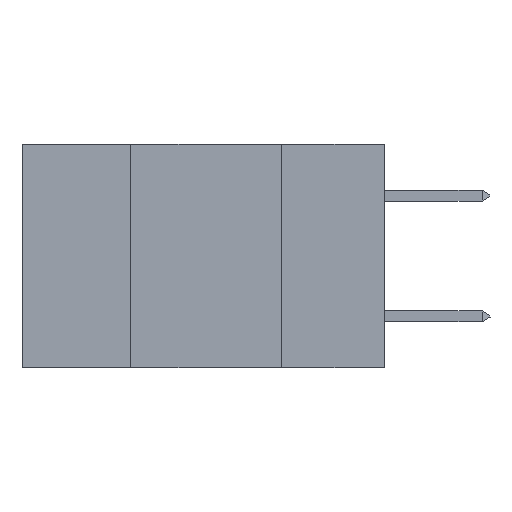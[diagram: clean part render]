
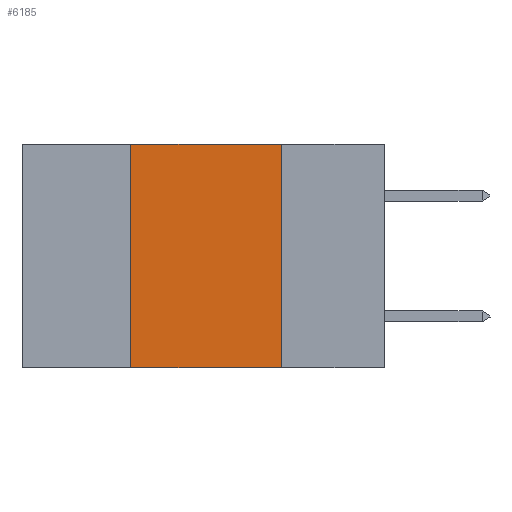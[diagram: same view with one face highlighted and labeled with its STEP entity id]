
A CAD part, left-side view. The second image highlights one B-rep face of the part: STEP entity #6185.
In plain terms, the highlighted planar face has unit normal (-1, 0, 0).
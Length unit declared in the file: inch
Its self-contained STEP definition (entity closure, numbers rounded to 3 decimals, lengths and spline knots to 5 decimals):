
#1363 = EDGE_CURVE ( 'NONE', #12753, #10109, #22118, .T. ) ;
#2100 = CARTESIAN_POINT ( 'NONE',  ( 0., 0.17, 0. ) ) ;
#2631 = DIRECTION ( 'NONE',  ( 1., 0., 0. ) ) ;
#4251 = VECTOR ( 'NONE', #13621, 39.37008 ) ;
#4387 = ORIENTED_EDGE ( 'NONE', *, *, #22126, .F. ) ;
#5815 = ORIENTED_EDGE ( 'NONE', *, *, #17179, .F. ) ;
#6185 = ADVANCED_FACE ( 'NONE', ( #22213 ), #7156, .F. ) ;
#7050 = DIRECTION ( 'NONE',  ( 0., -1., 0. ) ) ;
#7156 = PLANE ( 'NONE',  #24758 ) ;
#8880 = VERTEX_POINT ( 'NONE', #9145 ) ;
#9145 = CARTESIAN_POINT ( 'NONE',  ( 0., 0.42, 0. ) ) ;
#9714 = CARTESIAN_POINT ( 'NONE',  ( 0., 0.17, 0. ) ) ;
#10109 = VERTEX_POINT ( 'NONE', #13643 ) ;
#10728 = LINE ( 'NONE', #18353, #13745 ) ;
#11104 = CARTESIAN_POINT ( 'NONE',  ( 0., 0.6, -0.37 ) ) ;
#11514 = ORIENTED_EDGE ( 'NONE', *, *, #1363, .F. ) ;
#12753 = VERTEX_POINT ( 'NONE', #9714 ) ;
#13314 = VECTOR ( 'NONE', #19285, 39.37008 ) ;
#13621 = DIRECTION ( 'NONE',  ( 0., -1., 0. ) ) ;
#13643 = CARTESIAN_POINT ( 'NONE',  ( 0., 0.17, -0.37 ) ) ;
#13745 = VECTOR ( 'NONE', #27083, 39.37008 ) ;
#15365 = ORIENTED_EDGE ( 'NONE', *, *, #23207, .T. ) ;
#15604 = VECTOR ( 'NONE', #7050, 39.37008 ) ;
#17179 = EDGE_CURVE ( 'NONE', #8880, #12753, #18447, .T. ) ;
#18353 = CARTESIAN_POINT ( 'NONE',  ( 0., 0.42, 0. ) ) ;
#18447 = LINE ( 'NONE', #19902, #4251 ) ;
#19285 = DIRECTION ( 'NONE',  ( 0., 0., -1. ) ) ;
#19902 = CARTESIAN_POINT ( 'NONE',  ( 0., 0.6, 0. ) ) ;
#19925 = DIRECTION ( 'NONE',  ( 0., 0., -1. ) ) ;
#20006 = CARTESIAN_POINT ( 'NONE',  ( 0., 0.42, -0.37 ) ) ;
#20103 = CARTESIAN_POINT ( 'NONE',  ( 0., 0.6, 0. ) ) ;
#21374 = LINE ( 'NONE', #11104, #15604 ) ;
#22118 = LINE ( 'NONE', #2100, #13314 ) ;
#22126 = EDGE_CURVE ( 'NONE', #27155, #8880, #10728, .T. ) ;
#22213 = FACE_OUTER_BOUND ( 'NONE', #22413, .T. ) ;
#22413 = EDGE_LOOP ( 'NONE', ( #11514, #5815, #4387, #15365 ) ) ;
#23207 = EDGE_CURVE ( 'NONE', #27155, #10109, #21374, .T. ) ;
#24758 = AXIS2_PLACEMENT_3D ( 'NONE', #20103, #2631, #19925 ) ;
#27083 = DIRECTION ( 'NONE',  ( 0., 0., 1. ) ) ;
#27155 = VERTEX_POINT ( 'NONE', #20006 ) ;
